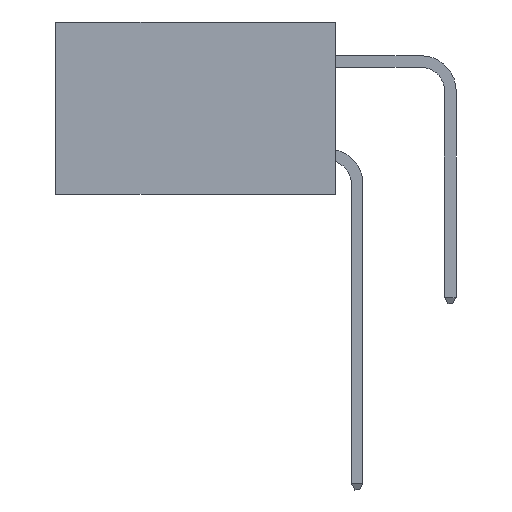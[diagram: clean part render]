
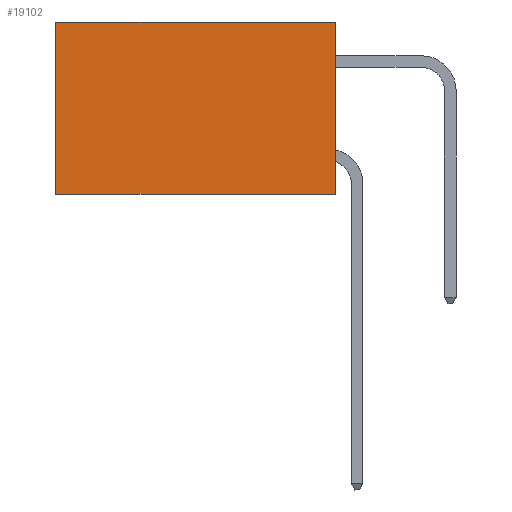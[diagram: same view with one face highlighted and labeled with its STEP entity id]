
A CAD part, left-side view. The second image highlights one B-rep face of the part: STEP entity #19102.
In plain terms, the highlighted planar face has unit normal (-1, 0, 0).
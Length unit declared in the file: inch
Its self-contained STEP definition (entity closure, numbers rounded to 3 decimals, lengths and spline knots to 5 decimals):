
#1140 = CARTESIAN_POINT ( 'NONE',  ( 0.2875, 0., 0. ) ) ;
#1172 = VECTOR ( 'NONE', #8599, 39.37008 ) ;
#2026 = FACE_OUTER_BOUND ( 'NONE', #20113, .T. ) ;
#2721 = PLANE ( 'NONE',  #17553 ) ;
#3713 = CARTESIAN_POINT ( 'NONE',  ( 0.2875, 0.6, 0. ) ) ;
#4346 = CARTESIAN_POINT ( 'NONE',  ( 0.2875, 0., -0.37 ) ) ;
#4586 = DIRECTION ( 'NONE',  ( 1., 0., 0. ) ) ;
#6466 = CARTESIAN_POINT ( 'NONE',  ( 0.2875, 0., 0. ) ) ;
#7256 = VERTEX_POINT ( 'NONE', #3713 ) ;
#7755 = VECTOR ( 'NONE', #9523, 39.37008 ) ;
#7995 = EDGE_CURVE ( 'NONE', #7256, #10828, #21026, .T. ) ;
#8131 = LINE ( 'NONE', #13313, #15588 ) ;
#8346 = DIRECTION ( 'NONE',  ( 0., 0., -1. ) ) ;
#8599 = DIRECTION ( 'NONE',  ( 0., 0., -1. ) ) ;
#8716 = ORIENTED_EDGE ( 'NONE', *, *, #23172, .F. ) ;
#8923 = ORIENTED_EDGE ( 'NONE', *, *, #7995, .T. ) ;
#9462 = EDGE_CURVE ( 'NONE', #13416, #10828, #19521, .T. ) ;
#9523 = DIRECTION ( 'NONE',  ( 0., 0., -1. ) ) ;
#10828 = VERTEX_POINT ( 'NONE', #21499 ) ;
#12620 = VECTOR ( 'NONE', #22930, 39.37008 ) ;
#13313 = CARTESIAN_POINT ( 'NONE',  ( 0.2875, 0., 0. ) ) ;
#13416 = VERTEX_POINT ( 'NONE', #21489 ) ;
#14929 = ORIENTED_EDGE ( 'NONE', *, *, #19535, .T. ) ;
#15109 = CARTESIAN_POINT ( 'NONE',  ( 0.2875, 0.6, 0. ) ) ;
#15588 = VECTOR ( 'NONE', #20647, 39.37008 ) ;
#17553 = AXIS2_PLACEMENT_3D ( 'NONE', #6466, #4586, #8346 ) ;
#19102 = ADVANCED_FACE ( 'NONE', ( #2026 ), #2721, .F. ) ;
#19521 = LINE ( 'NONE', #4346, #12620 ) ;
#19535 = EDGE_CURVE ( 'NONE', #21575, #7256, #8131, .T. ) ;
#19596 = CARTESIAN_POINT ( 'NONE',  ( 0.2875, 0., 0. ) ) ;
#20113 = EDGE_LOOP ( 'NONE', ( #8923, #21759, #8716, #14929 ) ) ;
#20274 = LINE ( 'NONE', #19596, #1172 ) ;
#20647 = DIRECTION ( 'NONE',  ( 0., 1., 0. ) ) ;
#21026 = LINE ( 'NONE', #15109, #7755 ) ;
#21489 = CARTESIAN_POINT ( 'NONE',  ( 0.2875, 0., -0.37 ) ) ;
#21499 = CARTESIAN_POINT ( 'NONE',  ( 0.2875, 0.6, -0.37 ) ) ;
#21575 = VERTEX_POINT ( 'NONE', #1140 ) ;
#21759 = ORIENTED_EDGE ( 'NONE', *, *, #9462, .F. ) ;
#22930 = DIRECTION ( 'NONE',  ( 0., 1., 0. ) ) ;
#23172 = EDGE_CURVE ( 'NONE', #21575, #13416, #20274, .T. ) ;
